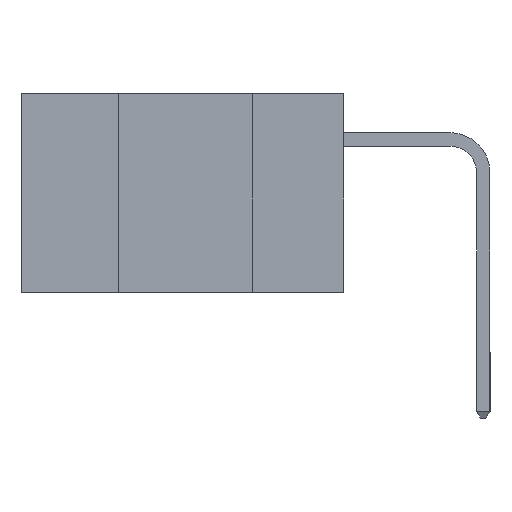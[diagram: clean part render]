
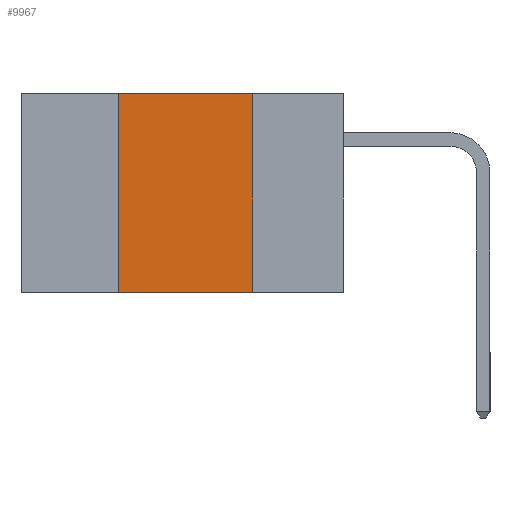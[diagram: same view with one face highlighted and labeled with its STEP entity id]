
A CAD part, left-side view. The second image highlights one B-rep face of the part: STEP entity #9967.
In plain terms, the highlighted planar face has unit normal (-1, 0, 0).
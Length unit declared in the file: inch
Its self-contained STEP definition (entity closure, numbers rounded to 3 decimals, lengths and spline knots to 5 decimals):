
#1311 = CARTESIAN_POINT ( 'NONE',  ( 0., 0.6, -0.37 ) ) ;
#1600 = VERTEX_POINT ( 'NONE', #11521 ) ;
#1688 = DIRECTION ( 'NONE',  ( 0., -1., 0. ) ) ;
#2165 = EDGE_LOOP ( 'NONE', ( #9865, #2833, #6851, #13393 ) ) ;
#2378 = EDGE_CURVE ( 'NONE', #8725, #14096, #6400, .T. ) ;
#2537 = LINE ( 'NONE', #12945, #15357 ) ;
#2833 = ORIENTED_EDGE ( 'NONE', *, *, #8856, .F. ) ;
#2903 = VECTOR ( 'NONE', #14214, 39.37008 ) ;
#2960 = CARTESIAN_POINT ( 'NONE',  ( 0., 0.17, -0.37 ) ) ;
#3283 = EDGE_CURVE ( 'NONE', #6647, #14096, #10249, .T. ) ;
#5206 = CARTESIAN_POINT ( 'NONE',  ( 0., 0.17, 0. ) ) ;
#6365 = PLANE ( 'NONE',  #14207 ) ;
#6400 = LINE ( 'NONE', #1311, #14894 ) ;
#6612 = LINE ( 'NONE', #11863, #7701 ) ;
#6647 = VERTEX_POINT ( 'NONE', #5206 ) ;
#6851 = ORIENTED_EDGE ( 'NONE', *, *, #15142, .F. ) ;
#7557 = DIRECTION ( 'NONE',  ( 0., 0., -1. ) ) ;
#7701 = VECTOR ( 'NONE', #1688, 39.37008 ) ;
#8725 = VERTEX_POINT ( 'NONE', #16537 ) ;
#8856 = EDGE_CURVE ( 'NONE', #1600, #6647, #6612, .T. ) ;
#9865 = ORIENTED_EDGE ( 'NONE', *, *, #3283, .F. ) ;
#9967 = ADVANCED_FACE ( 'NONE', ( #15427 ), #6365, .F. ) ;
#9998 = DIRECTION ( 'NONE',  ( 0., 0., 1. ) ) ;
#10249 = LINE ( 'NONE', #15410, #2903 ) ;
#10347 = DIRECTION ( 'NONE',  ( 1., 0., 0. ) ) ;
#11521 = CARTESIAN_POINT ( 'NONE',  ( 0., 0.42, 0. ) ) ;
#11564 = DIRECTION ( 'NONE',  ( 0., -1., 0. ) ) ;
#11863 = CARTESIAN_POINT ( 'NONE',  ( 0., 0.6, 0. ) ) ;
#12945 = CARTESIAN_POINT ( 'NONE',  ( 0., 0.42, -0.37 ) ) ;
#13393 = ORIENTED_EDGE ( 'NONE', *, *, #2378, .T. ) ;
#14096 = VERTEX_POINT ( 'NONE', #2960 ) ;
#14207 = AXIS2_PLACEMENT_3D ( 'NONE', #15502, #10347, #7557 ) ;
#14214 = DIRECTION ( 'NONE',  ( 0., 0., -1. ) ) ;
#14894 = VECTOR ( 'NONE', #11564, 39.37008 ) ;
#15142 = EDGE_CURVE ( 'NONE', #8725, #1600, #2537, .T. ) ;
#15357 = VECTOR ( 'NONE', #9998, 39.37008 ) ;
#15410 = CARTESIAN_POINT ( 'NONE',  ( 0., 0.17, -0.37 ) ) ;
#15427 = FACE_OUTER_BOUND ( 'NONE', #2165, .T. ) ;
#15502 = CARTESIAN_POINT ( 'NONE',  ( 0., 0.6, 0. ) ) ;
#16537 = CARTESIAN_POINT ( 'NONE',  ( 0., 0.42, -0.37 ) ) ;
